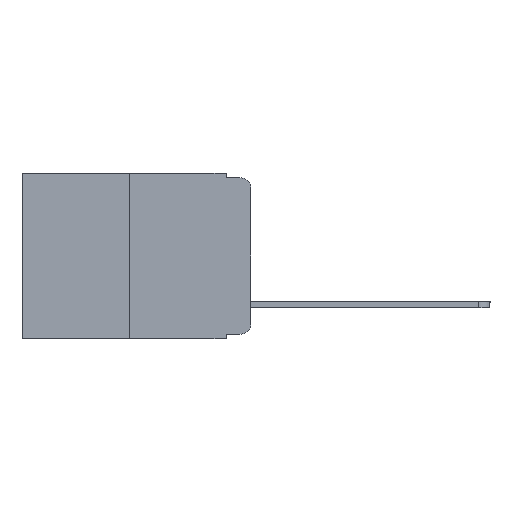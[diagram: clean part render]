
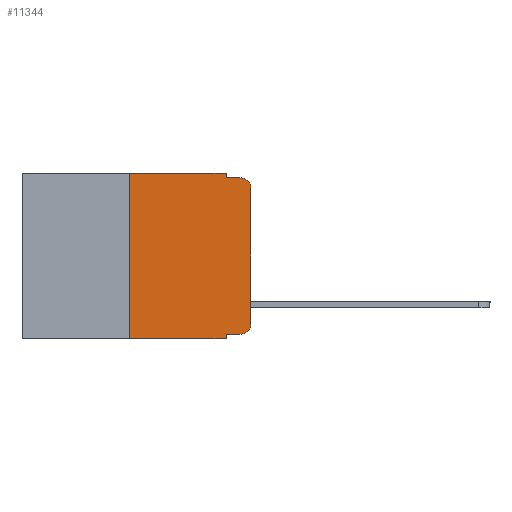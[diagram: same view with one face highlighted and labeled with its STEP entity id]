
A CAD part, left-side view. The second image highlights one B-rep face of the part: STEP entity #11344.
In plain terms, the highlighted planar face has unit normal (-1, 0, 0).
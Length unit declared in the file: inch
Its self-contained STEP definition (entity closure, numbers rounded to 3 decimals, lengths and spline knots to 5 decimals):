
#24 = ORIENTED_EDGE ( 'NONE', *, *, #3407, .F. ) ;
#39 = DIRECTION ( 'NONE',  ( 0., 0., -1. ) ) ;
#361 = DIRECTION ( 'NONE',  ( 0., 0., -1. ) ) ;
#444 = VECTOR ( 'NONE', #15538, 39.37008 ) ;
#484 = VECTOR ( 'NONE', #16266, 39.37008 ) ;
#516 = VECTOR ( 'NONE', #10515, 39.37008 ) ;
#600 = EDGE_CURVE ( 'NONE', #19074, #5884, #3013, .T. ) ;
#997 = CARTESIAN_POINT ( 'NONE',  ( 0., 0., -0.03 ) ) ;
#1062 = ORIENTED_EDGE ( 'NONE', *, *, #13231, .T. ) ;
#1173 = VERTEX_POINT ( 'NONE', #3693 ) ;
#1202 = CARTESIAN_POINT ( 'NONE',  ( 0., 0.051, -0.343 ) ) ;
#1369 = ORIENTED_EDGE ( 'NONE', *, *, #6579, .T. ) ;
#1594 = VECTOR ( 'NONE', #19816, 39.37008 ) ;
#1865 = DIRECTION ( 'NONE',  ( 0., -1., 0. ) ) ;
#2510 = LINE ( 'NONE', #17992, #13898 ) ;
#2522 = CARTESIAN_POINT ( 'NONE',  ( 0., 0.473, -0.343 ) ) ;
#2677 = FACE_OUTER_BOUND ( 'NONE', #12721, .T. ) ;
#2857 = VECTOR ( 'NONE', #15822, 39.37008 ) ;
#3013 = LINE ( 'NONE', #9266, #444 ) ;
#3266 = VERTEX_POINT ( 'NONE', #17294 ) ;
#3407 = EDGE_CURVE ( 'NONE', #16120, #3266, #2510, .T. ) ;
#3474 = ORIENTED_EDGE ( 'NONE', *, *, #14457, .T. ) ;
#3482 = DIRECTION ( 'NONE',  ( -1., 0., 0. ) ) ;
#3552 = LINE ( 'NONE', #3957, #484 ) ;
#3693 = CARTESIAN_POINT ( 'NONE',  ( 0., 0.02, -0.333 ) ) ;
#3957 = CARTESIAN_POINT ( 'NONE',  ( 0., 0.25, 0. ) ) ;
#4027 = CARTESIAN_POINT ( 'NONE',  ( 0., 0.02, -0.01 ) ) ;
#4232 = CARTESIAN_POINT ( 'NONE',  ( 0., 0.473, 0. ) ) ;
#4610 = EDGE_CURVE ( 'NONE', #4838, #16120, #3552, .T. ) ;
#4838 = VERTEX_POINT ( 'NONE', #15646 ) ;
#4920 = VERTEX_POINT ( 'NONE', #4970 ) ;
#4954 = CARTESIAN_POINT ( 'NONE',  ( 0., 0.051, -0.333 ) ) ;
#4970 = CARTESIAN_POINT ( 'NONE',  ( 0., 0.051, -0.01 ) ) ;
#5884 = VERTEX_POINT ( 'NONE', #997 ) ;
#6186 = CARTESIAN_POINT ( 'NONE',  ( 0., 0., -0.313 ) ) ;
#6272 = CARTESIAN_POINT ( 'NONE',  ( 0., 0.051, -0.01 ) ) ;
#6277 = CARTESIAN_POINT ( 'NONE',  ( 0., 0.051, -0.333 ) ) ;
#6579 = EDGE_CURVE ( 'NONE', #17787, #1173, #14292, .T. ) ;
#6887 = CIRCLE ( 'NONE', #11807, 0.02 ) ;
#7082 = PLANE ( 'NONE',  #15044 ) ;
#7104 = CARTESIAN_POINT ( 'NONE',  ( 0., 0.051, 0. ) ) ;
#7193 = CIRCLE ( 'NONE', #18651, 0.02 ) ;
#7824 = CARTESIAN_POINT ( 'NONE',  ( 0., 0.02, -0.313 ) ) ;
#8930 = DIRECTION ( 'NONE',  ( 1., 0., 0. ) ) ;
#9266 = CARTESIAN_POINT ( 'NONE',  ( 0., 0., 0. ) ) ;
#9680 = EDGE_CURVE ( 'NONE', #3266, #4920, #12029, .T. ) ;
#9734 = DIRECTION ( 'NONE',  ( 0., 0., -1. ) ) ;
#9753 = VERTEX_POINT ( 'NONE', #4027 ) ;
#10515 = DIRECTION ( 'NONE',  ( 0., -1., 0. ) ) ;
#10603 = VERTEX_POINT ( 'NONE', #1202 ) ;
#10707 = EDGE_CURVE ( 'NONE', #17787, #10603, #17469, .T. ) ;
#11344 = ADVANCED_FACE ( 'NONE', ( #2677 ), #7082, .F. ) ;
#11807 = AXIS2_PLACEMENT_3D ( 'NONE', #7824, #14105, #39 ) ;
#12029 = LINE ( 'NONE', #7104, #1594 ) ;
#12554 = EDGE_CURVE ( 'NONE', #5884, #9753, #7193, .T. ) ;
#12721 = EDGE_LOOP ( 'NONE', ( #13628, #15249, #14472, #19809, #24, #12849, #3474, #18739, #1369, #1062 ) ) ;
#12849 = ORIENTED_EDGE ( 'NONE', *, *, #4610, .F. ) ;
#13231 = EDGE_CURVE ( 'NONE', #1173, #19074, #6887, .T. ) ;
#13628 = ORIENTED_EDGE ( 'NONE', *, *, #600, .T. ) ;
#13898 = VECTOR ( 'NONE', #19526, 39.37008 ) ;
#13919 = CARTESIAN_POINT ( 'NONE',  ( 0., 0.25, 0. ) ) ;
#14105 = DIRECTION ( 'NONE',  ( -1., 0., 0. ) ) ;
#14292 = LINE ( 'NONE', #4954, #17520 ) ;
#14355 = VECTOR ( 'NONE', #361, 39.37008 ) ;
#14457 = EDGE_CURVE ( 'NONE', #4838, #10603, #18516, .T. ) ;
#14472 = ORIENTED_EDGE ( 'NONE', *, *, #16576, .F. ) ;
#15044 = AXIS2_PLACEMENT_3D ( 'NONE', #4232, #8930, #16837 ) ;
#15249 = ORIENTED_EDGE ( 'NONE', *, *, #12554, .T. ) ;
#15528 = LINE ( 'NONE', #6272, #2857 ) ;
#15538 = DIRECTION ( 'NONE',  ( 0., 0., 1. ) ) ;
#15646 = CARTESIAN_POINT ( 'NONE',  ( 0., 0.25, -0.343 ) ) ;
#15707 = CARTESIAN_POINT ( 'NONE',  ( 0., 0.02, -0.03 ) ) ;
#15822 = DIRECTION ( 'NONE',  ( 0., -1., 0. ) ) ;
#16120 = VERTEX_POINT ( 'NONE', #13919 ) ;
#16266 = DIRECTION ( 'NONE',  ( 0., 0., 1. ) ) ;
#16576 = EDGE_CURVE ( 'NONE', #4920, #9753, #15528, .T. ) ;
#16837 = DIRECTION ( 'NONE',  ( 0., 0., -1. ) ) ;
#17294 = CARTESIAN_POINT ( 'NONE',  ( 0., 0.051, 0. ) ) ;
#17469 = LINE ( 'NONE', #18705, #14355 ) ;
#17520 = VECTOR ( 'NONE', #1865, 39.37008 ) ;
#17787 = VERTEX_POINT ( 'NONE', #6277 ) ;
#17992 = CARTESIAN_POINT ( 'NONE',  ( 0., 0.473, 0. ) ) ;
#18516 = LINE ( 'NONE', #2522, #516 ) ;
#18651 = AXIS2_PLACEMENT_3D ( 'NONE', #15707, #3482, #9734 ) ;
#18705 = CARTESIAN_POINT ( 'NONE',  ( 0., 0.051, 0. ) ) ;
#18739 = ORIENTED_EDGE ( 'NONE', *, *, #10707, .F. ) ;
#19074 = VERTEX_POINT ( 'NONE', #6186 ) ;
#19526 = DIRECTION ( 'NONE',  ( 0., -1., 0. ) ) ;
#19809 = ORIENTED_EDGE ( 'NONE', *, *, #9680, .F. ) ;
#19816 = DIRECTION ( 'NONE',  ( 0., 0., -1. ) ) ;
